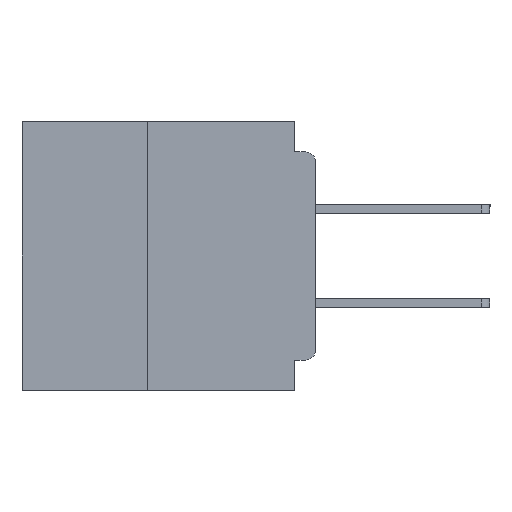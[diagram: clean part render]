
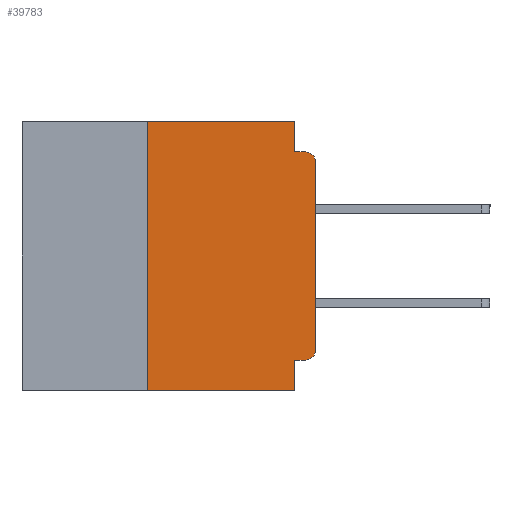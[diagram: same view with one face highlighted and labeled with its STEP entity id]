
A CAD part, left-side view. The second image highlights one B-rep face of the part: STEP entity #39783.
In plain terms, the highlighted planar face has unit normal (-1, 0, 0).
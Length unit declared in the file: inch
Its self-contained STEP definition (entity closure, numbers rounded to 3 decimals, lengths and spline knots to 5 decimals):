
#725 = ORIENTED_EDGE ( 'NONE', *, *, #39905, .F. ) ;
#2163 = EDGE_CURVE ( 'NONE', #33907, #36419, #41491, .T. ) ;
#2177 = LINE ( 'NONE', #27990, #32289 ) ;
#3748 = VECTOR ( 'NONE', #35626, 39.37008 ) ;
#4260 = CARTESIAN_POINT ( 'NONE',  ( 0., 0.015, -0.06 ) ) ;
#8066 = DIRECTION ( 'NONE',  ( 0., 0., -1. ) ) ;
#8697 = EDGE_LOOP ( 'NONE', ( #40725, #30430, #21666, #18258, #19565, #30903, #35564, #725, #37725, #35430 ) ) ;
#9166 = CARTESIAN_POINT ( 'NONE',  ( 0., 0.437, 0. ) ) ;
#9202 = EDGE_CURVE ( 'NONE', #15018, #23157, #31417, .T. ) ;
#10569 = AXIS2_PLACEMENT_3D ( 'NONE', #4260, #30663, #8066 ) ;
#10919 = AXIS2_PLACEMENT_3D ( 'NONE', #18893, #37854, #15221 ) ;
#10960 = VERTEX_POINT ( 'NONE', #24267 ) ;
#11266 = PLANE ( 'NONE',  #10919 ) ;
#12847 = VECTOR ( 'NONE', #42698, 39.37008 ) ;
#13531 = VERTEX_POINT ( 'NONE', #44966 ) ;
#15018 = VERTEX_POINT ( 'NONE', #38776 ) ;
#15185 = EDGE_CURVE ( 'NONE', #23157, #46522, #29500, .T. ) ;
#15221 = DIRECTION ( 'NONE',  ( 0., 0., -1. ) ) ;
#15871 = DIRECTION ( 'NONE',  ( 0., 0., -1. ) ) ;
#16051 = EDGE_CURVE ( 'NONE', #10960, #39152, #27068, .T. ) ;
#16731 = VECTOR ( 'NONE', #45558, 39.37008 ) ;
#16907 = DIRECTION ( 'NONE',  ( 0., -1., 0. ) ) ;
#17928 = LINE ( 'NONE', #23025, #16731 ) ;
#18258 = ORIENTED_EDGE ( 'NONE', *, *, #15185, .F. ) ;
#18893 = CARTESIAN_POINT ( 'NONE',  ( 0., 0.437, 0. ) ) ;
#19201 = CARTESIAN_POINT ( 'NONE',  ( 0., 0.031, 0. ) ) ;
#19475 = VECTOR ( 'NONE', #45515, 39.37008 ) ;
#19565 = ORIENTED_EDGE ( 'NONE', *, *, #9202, .F. ) ;
#19771 = AXIS2_PLACEMENT_3D ( 'NONE', #44631, #22073, #48358 ) ;
#20697 = DIRECTION ( 'NONE',  ( 0., 1., 0. ) ) ;
#21400 = VECTOR ( 'NONE', #16907, 39.37008 ) ;
#21666 = ORIENTED_EDGE ( 'NONE', *, *, #29318, .F. ) ;
#22073 = DIRECTION ( 'NONE',  ( -1., 0., 0. ) ) ;
#22629 = EDGE_CURVE ( 'NONE', #33907, #15018, #17928, .T. ) ;
#23025 = CARTESIAN_POINT ( 'NONE',  ( 0., 0.25, -0.4 ) ) ;
#23157 = VERTEX_POINT ( 'NONE', #34190 ) ;
#24267 = CARTESIAN_POINT ( 'NONE',  ( 0., 0.015, -0.355 ) ) ;
#27068 = LINE ( 'NONE', #43097, #45877 ) ;
#27723 = CARTESIAN_POINT ( 'NONE',  ( 0., 0., 0. ) ) ;
#27990 = CARTESIAN_POINT ( 'NONE',  ( 0., 0., -0.045 ) ) ;
#28042 = CARTESIAN_POINT ( 'NONE',  ( 0., 0.437, -0.4 ) ) ;
#28624 = EDGE_CURVE ( 'NONE', #13531, #33563, #32961, .T. ) ;
#29174 = CARTESIAN_POINT ( 'NONE',  ( 0., 0.25, -0.4 ) ) ;
#29318 = EDGE_CURVE ( 'NONE', #46522, #48298, #2177, .T. ) ;
#29451 = CARTESIAN_POINT ( 'NONE',  ( 0., 0.031, -0.4 ) ) ;
#29500 = LINE ( 'NONE', #19201, #19475 ) ;
#30430 = ORIENTED_EDGE ( 'NONE', *, *, #47766, .T. ) ;
#30663 = DIRECTION ( 'NONE',  ( -1., 0., 0. ) ) ;
#30714 = CIRCLE ( 'NONE', #10569, 0.015 ) ;
#30903 = ORIENTED_EDGE ( 'NONE', *, *, #22629, .F. ) ;
#31417 = LINE ( 'NONE', #9166, #21400 ) ;
#31496 = FACE_OUTER_BOUND ( 'NONE', #8697, .T. ) ;
#32289 = VECTOR ( 'NONE', #42969, 39.37008 ) ;
#32961 = LINE ( 'NONE', #27723, #12847 ) ;
#33563 = VERTEX_POINT ( 'NONE', #34635 ) ;
#33907 = VERTEX_POINT ( 'NONE', #29174 ) ;
#34190 = CARTESIAN_POINT ( 'NONE',  ( 0., 0.031, 0. ) ) ;
#34436 = VECTOR ( 'NONE', #15871, 39.37008 ) ;
#34635 = CARTESIAN_POINT ( 'NONE',  ( 0., 0., -0.06 ) ) ;
#35430 = ORIENTED_EDGE ( 'NONE', *, *, #48109, .T. ) ;
#35564 = ORIENTED_EDGE ( 'NONE', *, *, #2163, .T. ) ;
#35626 = DIRECTION ( 'NONE',  ( 0., -1., 0. ) ) ;
#36419 = VERTEX_POINT ( 'NONE', #29451 ) ;
#37725 = ORIENTED_EDGE ( 'NONE', *, *, #16051, .F. ) ;
#37854 = DIRECTION ( 'NONE',  ( 1., 0., 0. ) ) ;
#38493 = CARTESIAN_POINT ( 'NONE',  ( 0., 0.031, -0.4 ) ) ;
#38776 = CARTESIAN_POINT ( 'NONE',  ( 0., 0.25, 0. ) ) ;
#39152 = VERTEX_POINT ( 'NONE', #45271 ) ;
#39783 = ADVANCED_FACE ( 'NONE', ( #31496 ), #11266, .F. ) ;
#39905 = EDGE_CURVE ( 'NONE', #39152, #36419, #44438, .T. ) ;
#40725 = ORIENTED_EDGE ( 'NONE', *, *, #28624, .T. ) ;
#41491 = LINE ( 'NONE', #28042, #3748 ) ;
#42136 = CARTESIAN_POINT ( 'NONE',  ( 0., 0.015, -0.045 ) ) ;
#42698 = DIRECTION ( 'NONE',  ( 0., 0., 1. ) ) ;
#42969 = DIRECTION ( 'NONE',  ( 0., -1., 0. ) ) ;
#43097 = CARTESIAN_POINT ( 'NONE',  ( 0., 0., -0.355 ) ) ;
#43670 = CARTESIAN_POINT ( 'NONE',  ( 0., 0.031, -0.045 ) ) ;
#44438 = LINE ( 'NONE', #38493, #34436 ) ;
#44631 = CARTESIAN_POINT ( 'NONE',  ( 0., 0.015, -0.34 ) ) ;
#44966 = CARTESIAN_POINT ( 'NONE',  ( 0., 0., -0.34 ) ) ;
#45271 = CARTESIAN_POINT ( 'NONE',  ( 0., 0.031, -0.355 ) ) ;
#45375 = CIRCLE ( 'NONE', #19771, 0.015 ) ;
#45515 = DIRECTION ( 'NONE',  ( 0., 0., -1. ) ) ;
#45558 = DIRECTION ( 'NONE',  ( 0., 0., 1. ) ) ;
#45877 = VECTOR ( 'NONE', #20697, 39.37008 ) ;
#46522 = VERTEX_POINT ( 'NONE', #43670 ) ;
#47766 = EDGE_CURVE ( 'NONE', #33563, #48298, #30714, .T. ) ;
#48109 = EDGE_CURVE ( 'NONE', #10960, #13531, #45375, .T. ) ;
#48298 = VERTEX_POINT ( 'NONE', #42136 ) ;
#48358 = DIRECTION ( 'NONE',  ( 0., 0., -1. ) ) ;
